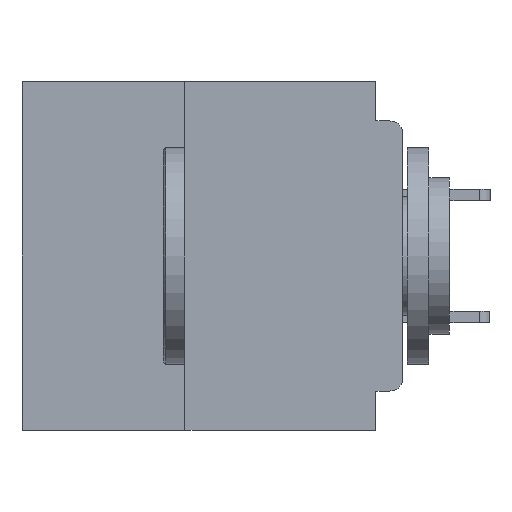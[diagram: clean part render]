
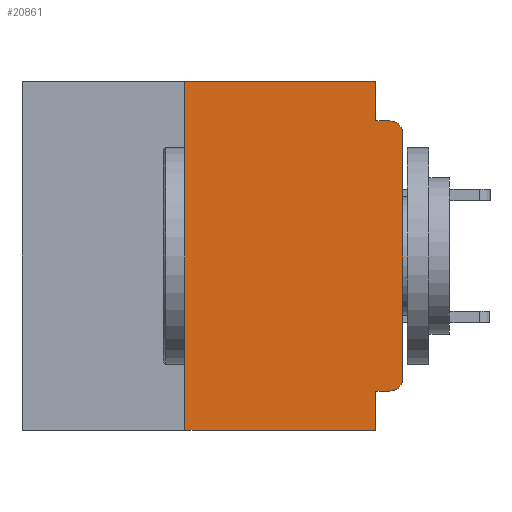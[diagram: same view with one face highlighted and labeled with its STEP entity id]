
A CAD part, left-side view. The second image highlights one B-rep face of the part: STEP entity #20861.
In plain terms, the highlighted planar face has unit normal (-1, 0, 0).
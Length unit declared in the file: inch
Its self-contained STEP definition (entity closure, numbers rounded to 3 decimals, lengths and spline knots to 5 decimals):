
#186 = ORIENTED_EDGE ( 'NONE', *, *, #4347, .T. ) ;
#1445 = ORIENTED_EDGE ( 'NONE', *, *, #33605, .F. ) ;
#1613 = ORIENTED_EDGE ( 'NONE', *, *, #36675, .F. ) ;
#1676 = PLANE ( 'NONE',  #32352 ) ;
#3037 = VECTOR ( 'NONE', #13199, 39.37008 ) ;
#4123 = LINE ( 'NONE', #33670, #3037 ) ;
#4347 = EDGE_CURVE ( 'NONE', #4607, #34027, #10687, .T. ) ;
#4607 = VERTEX_POINT ( 'NONE', #19526 ) ;
#4912 = CARTESIAN_POINT ( 'NONE',  ( 0., 0.25, -0.4 ) ) ;
#5275 = CARTESIAN_POINT ( 'NONE',  ( 0., 0.031, -0.4 ) ) ;
#5481 = EDGE_CURVE ( 'NONE', #8975, #37582, #6684, .T. ) ;
#5664 = ORIENTED_EDGE ( 'NONE', *, *, #16674, .T. ) ;
#5723 = AXIS2_PLACEMENT_3D ( 'NONE', #34150, #13704, #37517 ) ;
#6583 = CARTESIAN_POINT ( 'NONE',  ( 0., 0.031, 0. ) ) ;
#6631 = DIRECTION ( 'NONE',  ( 0., 0., 1. ) ) ;
#6684 = LINE ( 'NONE', #13750, #39868 ) ;
#6938 = VECTOR ( 'NONE', #42772, 39.37008 ) ;
#8533 = VERTEX_POINT ( 'NONE', #25896 ) ;
#8723 = CARTESIAN_POINT ( 'NONE',  ( 0., 0.437, 0. ) ) ;
#8975 = VERTEX_POINT ( 'NONE', #21327 ) ;
#10687 = LINE ( 'NONE', #41762, #11761 ) ;
#10738 = FACE_OUTER_BOUND ( 'NONE', #36183, .T. ) ;
#10951 = LINE ( 'NONE', #26989, #37125 ) ;
#11548 = EDGE_CURVE ( 'NONE', #27196, #8533, #10951, .T. ) ;
#11761 = VECTOR ( 'NONE', #21373, 39.37008 ) ;
#12026 = ORIENTED_EDGE ( 'NONE', *, *, #23168, .F. ) ;
#12298 = CARTESIAN_POINT ( 'NONE',  ( 0., 0., -0.045 ) ) ;
#12433 = VERTEX_POINT ( 'NONE', #28677 ) ;
#12906 = DIRECTION ( 'NONE',  ( 0., 1., 0. ) ) ;
#13199 = DIRECTION ( 'NONE',  ( 0., 0., -1. ) ) ;
#13704 = DIRECTION ( 'NONE',  ( -1., 0., 0. ) ) ;
#13750 = CARTESIAN_POINT ( 'NONE',  ( 0., 0.437, 0. ) ) ;
#14308 = DIRECTION ( 'NONE',  ( -1., 0., 0. ) ) ;
#15705 = DIRECTION ( 'NONE',  ( 1., 0., 0. ) ) ;
#16674 = EDGE_CURVE ( 'NONE', #36267, #4607, #18118, .T. ) ;
#17145 = ORIENTED_EDGE ( 'NONE', *, *, #5481, .F. ) ;
#17233 = DIRECTION ( 'NONE',  ( 0., -1., 0. ) ) ;
#17304 = LINE ( 'NONE', #5275, #6938 ) ;
#18118 = CIRCLE ( 'NONE', #37313, 0.015 ) ;
#18629 = CARTESIAN_POINT ( 'NONE',  ( 0., 0., -0.06 ) ) ;
#19519 = LINE ( 'NONE', #37472, #27558 ) ;
#19526 = CARTESIAN_POINT ( 'NONE',  ( 0., 0., -0.34 ) ) ;
#20098 = DIRECTION ( 'NONE',  ( 0., -1., 0. ) ) ;
#20759 = VERTEX_POINT ( 'NONE', #32258 ) ;
#20861 = ADVANCED_FACE ( 'NONE', ( #10738 ), #1676, .F. ) ;
#21327 = CARTESIAN_POINT ( 'NONE',  ( 0., 0.25, 0. ) ) ;
#21373 = DIRECTION ( 'NONE',  ( 0., 0., 1. ) ) ;
#22130 = ORIENTED_EDGE ( 'NONE', *, *, #11548, .T. ) ;
#23168 = EDGE_CURVE ( 'NONE', #36267, #20759, #23887, .T. ) ;
#23887 = LINE ( 'NONE', #33394, #41768 ) ;
#24917 = VECTOR ( 'NONE', #32807, 39.37008 ) ;
#25000 = EDGE_CURVE ( 'NONE', #37582, #27235, #4123, .T. ) ;
#25432 = ORIENTED_EDGE ( 'NONE', *, *, #30519, .T. ) ;
#25896 = CARTESIAN_POINT ( 'NONE',  ( 0., 0.031, -0.4 ) ) ;
#26989 = CARTESIAN_POINT ( 'NONE',  ( 0., 0.437, -0.4 ) ) ;
#27196 = VERTEX_POINT ( 'NONE', #4912 ) ;
#27235 = VERTEX_POINT ( 'NONE', #32736 ) ;
#27377 = CARTESIAN_POINT ( 'NONE',  ( 0., 0.015, -0.355 ) ) ;
#27558 = VECTOR ( 'NONE', #6631, 39.37008 ) ;
#27602 = ORIENTED_EDGE ( 'NONE', *, *, #25000, .F. ) ;
#28677 = CARTESIAN_POINT ( 'NONE',  ( 0., 0.015, -0.045 ) ) ;
#30519 = EDGE_CURVE ( 'NONE', #34027, #12433, #35107, .T. ) ;
#32165 = ORIENTED_EDGE ( 'NONE', *, *, #42813, .F. ) ;
#32258 = CARTESIAN_POINT ( 'NONE',  ( 0., 0.031, -0.355 ) ) ;
#32352 = AXIS2_PLACEMENT_3D ( 'NONE', #8723, #15705, #39468 ) ;
#32736 = CARTESIAN_POINT ( 'NONE',  ( 0., 0.031, -0.045 ) ) ;
#32791 = LINE ( 'NONE', #12298, #24917 ) ;
#32807 = DIRECTION ( 'NONE',  ( 0., -1., 0. ) ) ;
#33394 = CARTESIAN_POINT ( 'NONE',  ( 0., 0., -0.355 ) ) ;
#33605 = EDGE_CURVE ( 'NONE', #20759, #8533, #17304, .T. ) ;
#33670 = CARTESIAN_POINT ( 'NONE',  ( 0., 0.031, 0. ) ) ;
#34027 = VERTEX_POINT ( 'NONE', #18629 ) ;
#34150 = CARTESIAN_POINT ( 'NONE',  ( 0., 0.015, -0.06 ) ) ;
#34746 = CARTESIAN_POINT ( 'NONE',  ( 0., 0.015, -0.34 ) ) ;
#35107 = CIRCLE ( 'NONE', #5723, 0.015 ) ;
#36183 = EDGE_LOOP ( 'NONE', ( #186, #25432, #1613, #27602, #17145, #32165, #22130, #1445, #12026, #5664 ) ) ;
#36267 = VERTEX_POINT ( 'NONE', #27377 ) ;
#36675 = EDGE_CURVE ( 'NONE', #27235, #12433, #32791, .T. ) ;
#37125 = VECTOR ( 'NONE', #20098, 39.37008 ) ;
#37313 = AXIS2_PLACEMENT_3D ( 'NONE', #34746, #14308, #38112 ) ;
#37472 = CARTESIAN_POINT ( 'NONE',  ( 0., 0.25, -0.4 ) ) ;
#37517 = DIRECTION ( 'NONE',  ( 0., 0., -1. ) ) ;
#37582 = VERTEX_POINT ( 'NONE', #6583 ) ;
#38112 = DIRECTION ( 'NONE',  ( 0., 0., -1. ) ) ;
#39468 = DIRECTION ( 'NONE',  ( 0., 0., -1. ) ) ;
#39868 = VECTOR ( 'NONE', #17233, 39.37008 ) ;
#41762 = CARTESIAN_POINT ( 'NONE',  ( 0., 0., 0. ) ) ;
#41768 = VECTOR ( 'NONE', #12906, 39.37008 ) ;
#42772 = DIRECTION ( 'NONE',  ( 0., 0., -1. ) ) ;
#42813 = EDGE_CURVE ( 'NONE', #27196, #8975, #19519, .T. ) ;
